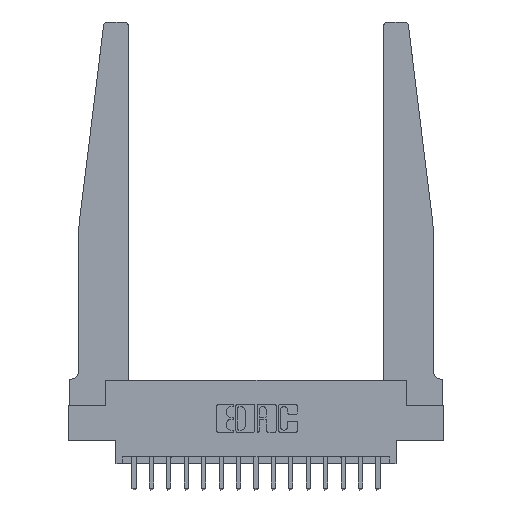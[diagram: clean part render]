
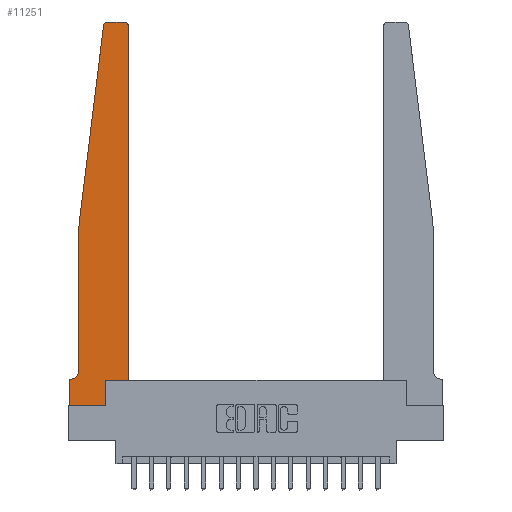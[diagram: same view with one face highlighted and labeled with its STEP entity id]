
A CAD part, top view. The second image highlights one B-rep face of the part: STEP entity #11251.
In plain terms, the highlighted planar face has unit normal (0, 0, 1).
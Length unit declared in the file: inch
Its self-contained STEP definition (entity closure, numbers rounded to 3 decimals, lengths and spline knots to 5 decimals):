
#9 = CARTESIAN_POINT ( 'NONE',  ( 0.425, 0.18, 0.37 ) ) ;
#104 = DIRECTION ( 'NONE',  ( -0.122, -0.992, 0. ) ) ;
#759 = LINE ( 'NONE', #8408, #15572 ) ;
#796 = VERTEX_POINT ( 'NONE', #10512 ) ;
#928 = VERTEX_POINT ( 'NONE', #17228 ) ;
#1371 = DIRECTION ( 'NONE',  ( 0., 1., 0. ) ) ;
#1420 = CARTESIAN_POINT ( 'NONE',  ( 0.27653, 2.75, 0.37 ) ) ;
#1545 = CARTESIAN_POINT ( 'NONE',  ( 0., 0., 0.37 ) ) ;
#1853 = VECTOR ( 'NONE', #2942, 39.37008 ) ;
#1906 = ORIENTED_EDGE ( 'NONE', *, *, #13860, .T. ) ;
#1935 = CARTESIAN_POINT ( 'NONE',  ( 0.065, 0.2375, 0.37 ) ) ;
#2033 = VECTOR ( 'NONE', #13037, 39.37008 ) ;
#2039 = ORIENTED_EDGE ( 'NONE', *, *, #14588, .T. ) ;
#2075 = CARTESIAN_POINT ( 'NONE',  ( 0.065, 1.25, 0.37 ) ) ;
#2081 = LINE ( 'NONE', #2075, #9328 ) ;
#2271 = DIRECTION ( 'NONE',  ( 0., 0., 1. ) ) ;
#2531 = CARTESIAN_POINT ( 'NONE',  ( 0.395, 2.75, 0.37 ) ) ;
#2766 = CARTESIAN_POINT ( 'NONE',  ( 0.015, 0.2375, 0.37 ) ) ;
#2942 = DIRECTION ( 'NONE',  ( 1., 0., 0. ) ) ;
#3170 = CIRCLE ( 'NONE', #17171, 0.03 ) ;
#3243 = CARTESIAN_POINT ( 'NONE',  ( 0.425, 0.18, 0.37 ) ) ;
#3736 = DIRECTION ( 'NONE',  ( 0., 0., 1. ) ) ;
#4187 = CARTESIAN_POINT ( 'NONE',  ( 0.425, 0.18, 0.37 ) ) ;
#4191 = DIRECTION ( 'NONE',  ( -1., 0., 0. ) ) ;
#4396 = CARTESIAN_POINT ( 'NONE',  ( 0.24675, 2.72367, 0.37 ) ) ;
#4418 = VECTOR ( 'NONE', #104, 39.37008 ) ;
#4545 = VERTEX_POINT ( 'NONE', #16458 ) ;
#4680 = AXIS2_PLACEMENT_3D ( 'NONE', #2766, #12849, #4191 ) ;
#4687 = ORIENTED_EDGE ( 'NONE', *, *, #5410, .T. ) ;
#5286 = LINE ( 'NONE', #17508, #12515 ) ;
#5410 = EDGE_CURVE ( 'NONE', #11923, #11408, #8542, .T. ) ;
#5515 = DIRECTION ( 'NONE',  ( 0., 1., 0. ) ) ;
#5782 = EDGE_LOOP ( 'NONE', ( #8193, #18170, #7519, #6614, #2039, #7712, #13873, #8391, #4687, #12384, #6464, #1906 ) ) ;
#6146 = CARTESIAN_POINT ( 'NONE',  ( 0.425, 2.72, 0.37 ) ) ;
#6440 = CARTESIAN_POINT ( 'NONE',  ( 0., 0., 0.37 ) ) ;
#6464 = ORIENTED_EDGE ( 'NONE', *, *, #11932, .T. ) ;
#6614 = ORIENTED_EDGE ( 'NONE', *, *, #13246, .T. ) ;
#6672 = CIRCLE ( 'NONE', #14201, 0.03 ) ;
#6734 = VERTEX_POINT ( 'NONE', #1545 ) ;
#6875 = DIRECTION ( 'NONE',  ( 0., 0., 1. ) ) ;
#6958 = AXIS2_PLACEMENT_3D ( 'NONE', #12513, #6875, #16726 ) ;
#7134 = EDGE_CURVE ( 'NONE', #928, #796, #5286, .T. ) ;
#7404 = VERTEX_POINT ( 'NONE', #2531 ) ;
#7519 = ORIENTED_EDGE ( 'NONE', *, *, #9432, .T. ) ;
#7712 = ORIENTED_EDGE ( 'NONE', *, *, #7134, .T. ) ;
#7858 = EDGE_CURVE ( 'NONE', #6734, #11923, #16805, .T. ) ;
#7915 = DIRECTION ( 'NONE',  ( 1., 0., 0. ) ) ;
#8193 = ORIENTED_EDGE ( 'NONE', *, *, #14636, .T. ) ;
#8249 = PLANE ( 'NONE',  #6958 ) ;
#8378 = VERTEX_POINT ( 'NONE', #1935 ) ;
#8391 = ORIENTED_EDGE ( 'NONE', *, *, #7858, .T. ) ;
#8408 = CARTESIAN_POINT ( 'NONE',  ( 0., 0., 0.37 ) ) ;
#8542 = LINE ( 'NONE', #12752, #15634 ) ;
#8600 = CARTESIAN_POINT ( 'NONE',  ( 0.2605, 0., 0.37 ) ) ;
#8788 = CARTESIAN_POINT ( 'NONE',  ( 0.065, 1.25, 0.37 ) ) ;
#9328 = VECTOR ( 'NONE', #14990, 39.37008 ) ;
#9432 = EDGE_CURVE ( 'NONE', #17134, #4545, #10813, .T. ) ;
#9744 = LINE ( 'NONE', #17012, #2033 ) ;
#10030 = CARTESIAN_POINT ( 'NONE',  ( 0.2605, 0.18, 0.37 ) ) ;
#10512 = CARTESIAN_POINT ( 'NONE',  ( 0., 0.1875, 0.37 ) ) ;
#10793 = VERTEX_POINT ( 'NONE', #1420 ) ;
#10813 = LINE ( 'NONE', #8788, #4418 ) ;
#10957 = CARTESIAN_POINT ( 'NONE',  ( 0.27653, 2.72, 0.37 ) ) ;
#11251 = ADVANCED_FACE ( 'NONE', ( #14063 ), #8249, .T. ) ;
#11321 = DIRECTION ( 'NONE',  ( 0., -1., 0. ) ) ;
#11408 = VERTEX_POINT ( 'NONE', #10030 ) ;
#11821 = EDGE_CURVE ( 'NONE', #796, #6734, #759, .T. ) ;
#11923 = VERTEX_POINT ( 'NONE', #8600 ) ;
#11932 = EDGE_CURVE ( 'NONE', #13640, #14240, #14694, .T. ) ;
#12360 = DIRECTION ( 'NONE',  ( 1., 0., 0. ) ) ;
#12384 = ORIENTED_EDGE ( 'NONE', *, *, #13483, .T. ) ;
#12385 = CARTESIAN_POINT ( 'NONE',  ( 0.395, 2.72, 0.37 ) ) ;
#12513 = CARTESIAN_POINT ( 'NONE',  ( 0., 0.1875, 0.37 ) ) ;
#12515 = VECTOR ( 'NONE', #16134, 39.37008 ) ;
#12704 = VECTOR ( 'NONE', #7915, 39.37008 ) ;
#12752 = CARTESIAN_POINT ( 'NONE',  ( 0.2605, 0.18, 0.37 ) ) ;
#12849 = DIRECTION ( 'NONE',  ( 0., 0., -1. ) ) ;
#13037 = DIRECTION ( 'NONE',  ( -1., 0., 0. ) ) ;
#13246 = EDGE_CURVE ( 'NONE', #4545, #8378, #2081, .T. ) ;
#13330 = LINE ( 'NONE', #9, #1853 ) ;
#13483 = EDGE_CURVE ( 'NONE', #11408, #13640, #13330, .T. ) ;
#13640 = VERTEX_POINT ( 'NONE', #3243 ) ;
#13811 = DIRECTION ( 'NONE',  ( 1., 0., 0. ) ) ;
#13860 = EDGE_CURVE ( 'NONE', #14240, #7404, #3170, .T. ) ;
#13873 = ORIENTED_EDGE ( 'NONE', *, *, #11821, .T. ) ;
#13948 = CIRCLE ( 'NONE', #4680, 0.05 ) ;
#14063 = FACE_OUTER_BOUND ( 'NONE', #5782, .T. ) ;
#14201 = AXIS2_PLACEMENT_3D ( 'NONE', #10957, #2271, #12360 ) ;
#14240 = VERTEX_POINT ( 'NONE', #6146 ) ;
#14251 = VECTOR ( 'NONE', #1371, 39.37008 ) ;
#14588 = EDGE_CURVE ( 'NONE', #8378, #928, #13948, .T. ) ;
#14636 = EDGE_CURVE ( 'NONE', #7404, #10793, #9744, .T. ) ;
#14694 = LINE ( 'NONE', #4187, #14251 ) ;
#14990 = DIRECTION ( 'NONE',  ( 0., -1., 0. ) ) ;
#15572 = VECTOR ( 'NONE', #11321, 39.37008 ) ;
#15634 = VECTOR ( 'NONE', #5515, 39.37008 ) ;
#15793 = EDGE_CURVE ( 'NONE', #10793, #17134, #6672, .T. ) ;
#16134 = DIRECTION ( 'NONE',  ( -1., 0., 0. ) ) ;
#16458 = CARTESIAN_POINT ( 'NONE',  ( 0.065, 1.25, 0.37 ) ) ;
#16726 = DIRECTION ( 'NONE',  ( 1., 0., 0. ) ) ;
#16805 = LINE ( 'NONE', #6440, #12704 ) ;
#17012 = CARTESIAN_POINT ( 'NONE',  ( 0.25, 2.75, 0.37 ) ) ;
#17134 = VERTEX_POINT ( 'NONE', #4396 ) ;
#17171 = AXIS2_PLACEMENT_3D ( 'NONE', #12385, #3736, #13811 ) ;
#17228 = CARTESIAN_POINT ( 'NONE',  ( 0.015, 0.1875, 0.37 ) ) ;
#17508 = CARTESIAN_POINT ( 'NONE',  ( 0.065, 0.1875, 0.37 ) ) ;
#18170 = ORIENTED_EDGE ( 'NONE', *, *, #15793, .T. ) ;
